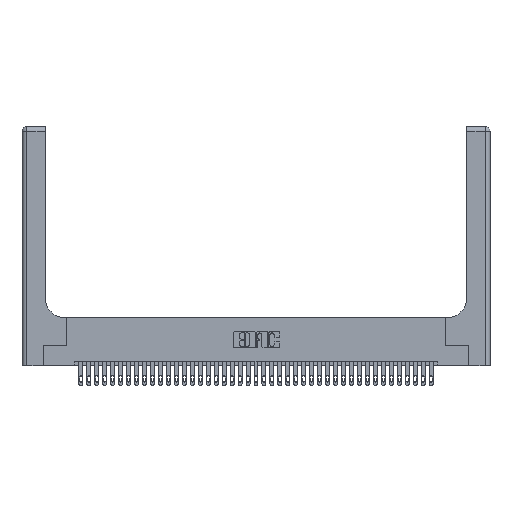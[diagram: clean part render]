
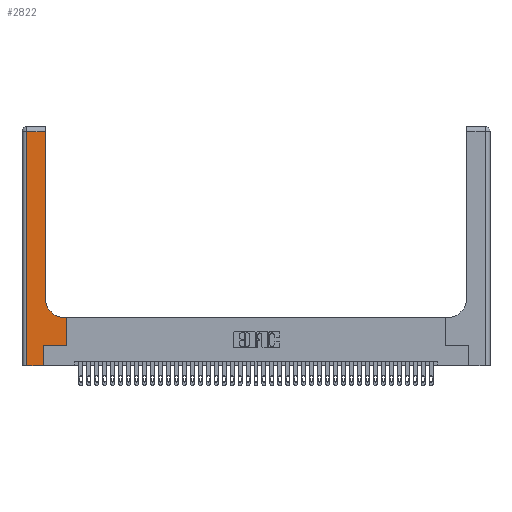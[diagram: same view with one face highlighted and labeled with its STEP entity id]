
A CAD part, top view. The second image highlights one B-rep face of the part: STEP entity #2822.
In plain terms, the highlighted planar face has unit normal (0, 0, 1).
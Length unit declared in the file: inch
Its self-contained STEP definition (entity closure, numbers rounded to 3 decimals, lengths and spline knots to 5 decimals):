
#503 = EDGE_CURVE ( 'NONE', #1471, #16858, #4446, .T. ) ;
#602 = CARTESIAN_POINT ( 'NONE',  ( 0.2915, 2.94, 0.37 ) ) ;
#1153 = ORIENTED_EDGE ( 'NONE', *, *, #17916, .T. ) ;
#1471 = VERTEX_POINT ( 'NONE', #29467 ) ;
#2348 = VERTEX_POINT ( 'NONE', #13123 ) ;
#2744 = VERTEX_POINT ( 'NONE', #13039 ) ;
#2822 = ADVANCED_FACE ( 'NONE', ( #9736 ), #21602, .F. ) ;
#2906 = LINE ( 'NONE', #29316, #15467 ) ;
#3361 = ORIENTED_EDGE ( 'NONE', *, *, #30114, .T. ) ;
#3368 = EDGE_CURVE ( 'NONE', #2348, #35512, #2906, .T. ) ;
#3489 = AXIS2_PLACEMENT_3D ( 'NONE', #30883, #37598, #24011 ) ;
#3660 = EDGE_CURVE ( 'NONE', #35512, #32647, #22694, .T. ) ;
#3833 = ORIENTED_EDGE ( 'NONE', *, *, #14552, .T. ) ;
#3995 = DIRECTION ( 'NONE',  ( -1., 0., 0. ) ) ;
#4038 = DIRECTION ( 'NONE',  ( -1., 0., 0. ) ) ;
#4446 = LINE ( 'NONE', #14868, #7853 ) ;
#5262 = VECTOR ( 'NONE', #27954, 39.37008 ) ;
#5877 = AXIS2_PLACEMENT_3D ( 'NONE', #6858, #18758, #34530 ) ;
#6184 = ORIENTED_EDGE ( 'NONE', *, *, #3368, .T. ) ;
#6858 = CARTESIAN_POINT ( 'NONE',  ( 0.5415, 0.85, 0.37 ) ) ;
#7487 = CARTESIAN_POINT ( 'NONE',  ( 0.06, 0., 0.37 ) ) ;
#7853 = VECTOR ( 'NONE', #32988, 39.37008 ) ;
#9736 = FACE_OUTER_BOUND ( 'NONE', #34212, .T. ) ;
#11043 = DIRECTION ( 'NONE',  ( 0., 1., 0. ) ) ;
#12171 = VERTEX_POINT ( 'NONE', #32282 ) ;
#13039 = CARTESIAN_POINT ( 'NONE',  ( 0.5585, 0.25, 0.37 ) ) ;
#13123 = CARTESIAN_POINT ( 'NONE',  ( 0.5585, 0.6, 0.37 ) ) ;
#14461 = VECTOR ( 'NONE', #19862, 39.37008 ) ;
#14552 = EDGE_CURVE ( 'NONE', #32647, #16076, #14959, .T. ) ;
#14675 = VECTOR ( 'NONE', #19446, 39.37008 ) ;
#14868 = CARTESIAN_POINT ( 'NONE',  ( 0.06, 3., 0.37 ) ) ;
#14959 = LINE ( 'NONE', #36776, #5262 ) ;
#15467 = VECTOR ( 'NONE', #4038, 39.37008 ) ;
#16076 = VERTEX_POINT ( 'NONE', #602 ) ;
#16858 = VERTEX_POINT ( 'NONE', #7487 ) ;
#17089 = ORIENTED_EDGE ( 'NONE', *, *, #28112, .T. ) ;
#17916 = EDGE_CURVE ( 'NONE', #2744, #2348, #34913, .T. ) ;
#18321 = EDGE_CURVE ( 'NONE', #12171, #36048, #28059, .T. ) ;
#18507 = VECTOR ( 'NONE', #27518, 39.37008 ) ;
#18758 = DIRECTION ( 'NONE',  ( 0., 0., -1. ) ) ;
#18918 = CARTESIAN_POINT ( 'NONE',  ( 0.269, 0.25, 0.37 ) ) ;
#19070 = ORIENTED_EDGE ( 'NONE', *, *, #32472, .T. ) ;
#19446 = DIRECTION ( 'NONE',  ( 1., 0., 0. ) ) ;
#19862 = DIRECTION ( 'NONE',  ( 1., 0., 0. ) ) ;
#20830 = CARTESIAN_POINT ( 'NONE',  ( 0.5415, 0.6, 0.37 ) ) ;
#21187 = ORIENTED_EDGE ( 'NONE', *, *, #503, .T. ) ;
#21602 = PLANE ( 'NONE',  #3489 ) ;
#22025 = VECTOR ( 'NONE', #3995, 39.37008 ) ;
#22381 = CARTESIAN_POINT ( 'NONE',  ( 0., 2.94, 0.37 ) ) ;
#22694 = CIRCLE ( 'NONE', #5877, 0.25 ) ;
#23001 = LINE ( 'NONE', #22381, #22025 ) ;
#24011 = DIRECTION ( 'NONE',  ( -1., 0., 0. ) ) ;
#26801 = CARTESIAN_POINT ( 'NONE',  ( 0.269, 0.25, 0.37 ) ) ;
#27084 = CARTESIAN_POINT ( 'NONE',  ( 0.2915, 0.85, 0.37 ) ) ;
#27518 = DIRECTION ( 'NONE',  ( 0., 1., 0. ) ) ;
#27945 = LINE ( 'NONE', #18918, #14461 ) ;
#27954 = DIRECTION ( 'NONE',  ( 0., 1., 0. ) ) ;
#28059 = LINE ( 'NONE', #29407, #30995 ) ;
#28112 = EDGE_CURVE ( 'NONE', #16076, #1471, #23001, .T. ) ;
#29316 = CARTESIAN_POINT ( 'NONE',  ( 0.2915, 0.6, 0.37 ) ) ;
#29407 = CARTESIAN_POINT ( 'NONE',  ( 0.269, 0., 0.37 ) ) ;
#29467 = CARTESIAN_POINT ( 'NONE',  ( 0.06, 2.94, 0.37 ) ) ;
#30114 = EDGE_CURVE ( 'NONE', #16858, #12171, #34473, .T. ) ;
#30883 = CARTESIAN_POINT ( 'NONE',  ( 0., 3., 0.37 ) ) ;
#30995 = VECTOR ( 'NONE', #11043, 39.37008 ) ;
#32282 = CARTESIAN_POINT ( 'NONE',  ( 0.269, 0., 0.37 ) ) ;
#32472 = EDGE_CURVE ( 'NONE', #36048, #2744, #27945, .T. ) ;
#32647 = VERTEX_POINT ( 'NONE', #27084 ) ;
#32988 = DIRECTION ( 'NONE',  ( 0., -1., 0. ) ) ;
#34212 = EDGE_LOOP ( 'NONE', ( #3833, #17089, #21187, #3361, #39078, #19070, #1153, #6184, #37863 ) ) ;
#34473 = LINE ( 'NONE', #37951, #14675 ) ;
#34530 = DIRECTION ( 'NONE',  ( 1., 0., 0. ) ) ;
#34913 = LINE ( 'NONE', #36461, #18507 ) ;
#35512 = VERTEX_POINT ( 'NONE', #20830 ) ;
#36048 = VERTEX_POINT ( 'NONE', #26801 ) ;
#36461 = CARTESIAN_POINT ( 'NONE',  ( 0.5585, 0.25, 0.37 ) ) ;
#36776 = CARTESIAN_POINT ( 'NONE',  ( 0.2915, 3., 0.37 ) ) ;
#37598 = DIRECTION ( 'NONE',  ( 0., 0., -1. ) ) ;
#37863 = ORIENTED_EDGE ( 'NONE', *, *, #3660, .T. ) ;
#37951 = CARTESIAN_POINT ( 'NONE',  ( 0., 0., 0.37 ) ) ;
#39078 = ORIENTED_EDGE ( 'NONE', *, *, #18321, .T. ) ;
